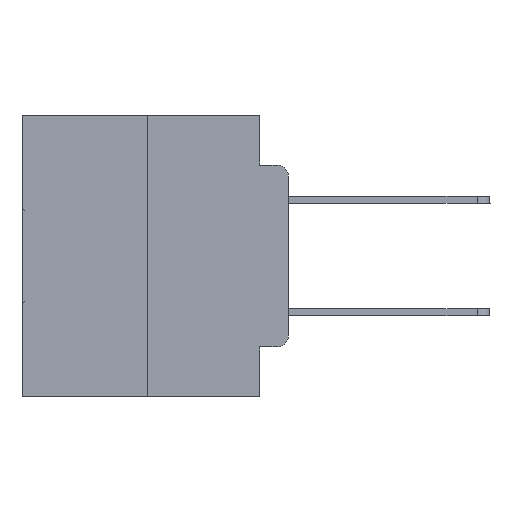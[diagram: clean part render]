
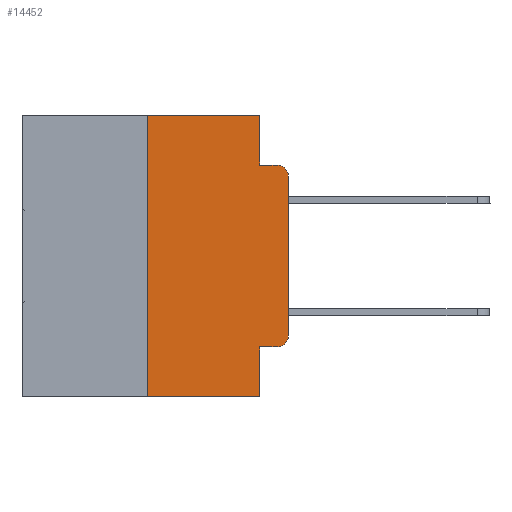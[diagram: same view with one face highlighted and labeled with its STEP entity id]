
A CAD part, left-side view. The second image highlights one B-rep face of the part: STEP entity #14452.
In plain terms, the highlighted planar face has unit normal (-1, 0, 0).
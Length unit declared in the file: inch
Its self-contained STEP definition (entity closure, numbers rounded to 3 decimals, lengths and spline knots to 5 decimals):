
#887 = VECTOR ( 'NONE', #26429, 39.37008 ) ;
#1592 = CARTESIAN_POINT ( 'NONE',  ( 0., 0.051, -0.0885 ) ) ;
#2279 = DIRECTION ( 'NONE',  ( 0., 0., -1. ) ) ;
#2426 = DIRECTION ( 'NONE',  ( 0., 0., 1. ) ) ;
#2488 = VERTEX_POINT ( 'NONE', #21263 ) ;
#2617 = AXIS2_PLACEMENT_3D ( 'NONE', #30579, #9293, #16163 ) ;
#2816 = ORIENTED_EDGE ( 'NONE', *, *, #7497, .T. ) ;
#3326 = CARTESIAN_POINT ( 'NONE',  ( 0., 0.25, 0. ) ) ;
#3633 = VERTEX_POINT ( 'NONE', #7026 ) ;
#3906 = VERTEX_POINT ( 'NONE', #6482 ) ;
#5116 = EDGE_CURVE ( 'NONE', #2488, #24602, #30207, .T. ) ;
#5413 = DIRECTION ( 'NONE',  ( 0., 0., 1. ) ) ;
#5499 = VERTEX_POINT ( 'NONE', #8828 ) ;
#6482 = CARTESIAN_POINT ( 'NONE',  ( 0., 0.051, -0.4115 ) ) ;
#6509 = VECTOR ( 'NONE', #29588, 39.37008 ) ;
#7026 = CARTESIAN_POINT ( 'NONE',  ( 0., 0., -0.1085 ) ) ;
#7497 = EDGE_CURVE ( 'NONE', #2488, #29429, #12756, .T. ) ;
#7513 = CARTESIAN_POINT ( 'NONE',  ( 0., 0.051, -0.5 ) ) ;
#8701 = AXIS2_PLACEMENT_3D ( 'NONE', #16530, #21446, #2279 ) ;
#8759 = CARTESIAN_POINT ( 'NONE',  ( 0., 0.051, -0.0885 ) ) ;
#8828 = CARTESIAN_POINT ( 'NONE',  ( 0., 0., -0.3915 ) ) ;
#9293 = DIRECTION ( 'NONE',  ( 1., 0., 0. ) ) ;
#9789 = VECTOR ( 'NONE', #5413, 39.37008 ) ;
#10036 = ORIENTED_EDGE ( 'NONE', *, *, #5116, .F. ) ;
#10191 = VERTEX_POINT ( 'NONE', #1592 ) ;
#10495 = VECTOR ( 'NONE', #16469, 39.37008 ) ;
#10659 = VERTEX_POINT ( 'NONE', #20377 ) ;
#10724 = LINE ( 'NONE', #8759, #15228 ) ;
#12074 = DIRECTION ( 'NONE',  ( 0., 0., -1. ) ) ;
#12575 = LINE ( 'NONE', #21474, #887 ) ;
#12756 = LINE ( 'NONE', #31098, #10495 ) ;
#12823 = CARTESIAN_POINT ( 'NONE',  ( 0., 0.473, 0. ) ) ;
#12904 = LINE ( 'NONE', #12823, #6509 ) ;
#12958 = EDGE_CURVE ( 'NONE', #24602, #29509, #12904, .T. ) ;
#13052 = DIRECTION ( 'NONE',  ( 0., 0., -1. ) ) ;
#13186 = FACE_OUTER_BOUND ( 'NONE', #17552, .T. ) ;
#13832 = EDGE_CURVE ( 'NONE', #14276, #5499, #26831, .T. ) ;
#14136 = VECTOR ( 'NONE', #13052, 39.37008 ) ;
#14276 = VERTEX_POINT ( 'NONE', #27922 ) ;
#14342 = CARTESIAN_POINT ( 'NONE',  ( 0., 0.25, 0. ) ) ;
#14365 = DIRECTION ( 'NONE',  ( 0., 0., -1. ) ) ;
#14381 = DIRECTION ( 'NONE',  ( -1., 0., 0. ) ) ;
#14452 = ADVANCED_FACE ( 'NONE', ( #13186 ), #30798, .F. ) ;
#14622 = EDGE_CURVE ( 'NONE', #5499, #3633, #23374, .T. ) ;
#15228 = VECTOR ( 'NONE', #23198, 39.37008 ) ;
#15565 = ORIENTED_EDGE ( 'NONE', *, *, #13832, .T. ) ;
#16163 = DIRECTION ( 'NONE',  ( 0., 0., -1. ) ) ;
#16469 = DIRECTION ( 'NONE',  ( 0., -1., 0. ) ) ;
#16530 = CARTESIAN_POINT ( 'NONE',  ( 0., 0.02, -0.1085 ) ) ;
#17552 = EDGE_LOOP ( 'NONE', ( #24741, #29118, #23249, #23381, #22470, #10036, #2816, #29877, #19213, #15565 ) ) ;
#17888 = LINE ( 'NONE', #29405, #14136 ) ;
#19213 = ORIENTED_EDGE ( 'NONE', *, *, #25050, .T. ) ;
#20377 = CARTESIAN_POINT ( 'NONE',  ( 0., 0.02, -0.0885 ) ) ;
#21263 = CARTESIAN_POINT ( 'NONE',  ( 0., 0.25, -0.5 ) ) ;
#21446 = DIRECTION ( 'NONE',  ( -1., 0., 0. ) ) ;
#21474 = CARTESIAN_POINT ( 'NONE',  ( 0., 0.051, -0.4115 ) ) ;
#21711 = EDGE_CURVE ( 'NONE', #29509, #10191, #31122, .T. ) ;
#21881 = EDGE_CURVE ( 'NONE', #3906, #29429, #17888, .T. ) ;
#22470 = ORIENTED_EDGE ( 'NONE', *, *, #12958, .F. ) ;
#23011 = EDGE_CURVE ( 'NONE', #3633, #10659, #29554, .T. ) ;
#23023 = VECTOR ( 'NONE', #2426, 39.37008 ) ;
#23198 = DIRECTION ( 'NONE',  ( 0., -1., 0. ) ) ;
#23249 = ORIENTED_EDGE ( 'NONE', *, *, #24182, .F. ) ;
#23374 = LINE ( 'NONE', #31200, #9789 ) ;
#23381 = ORIENTED_EDGE ( 'NONE', *, *, #21711, .F. ) ;
#23590 = VECTOR ( 'NONE', #14365, 39.37008 ) ;
#23960 = CARTESIAN_POINT ( 'NONE',  ( 0., 0.02, -0.3915 ) ) ;
#24046 = CARTESIAN_POINT ( 'NONE',  ( 0., 0.051, 0. ) ) ;
#24182 = EDGE_CURVE ( 'NONE', #10191, #10659, #10724, .T. ) ;
#24589 = CARTESIAN_POINT ( 'NONE',  ( 0., 0.051, 0. ) ) ;
#24602 = VERTEX_POINT ( 'NONE', #3326 ) ;
#24608 = AXIS2_PLACEMENT_3D ( 'NONE', #23960, #14381, #12074 ) ;
#24741 = ORIENTED_EDGE ( 'NONE', *, *, #14622, .T. ) ;
#25050 = EDGE_CURVE ( 'NONE', #3906, #14276, #12575, .T. ) ;
#26429 = DIRECTION ( 'NONE',  ( 0., -1., 0. ) ) ;
#26831 = CIRCLE ( 'NONE', #24608, 0.02 ) ;
#27922 = CARTESIAN_POINT ( 'NONE',  ( 0., 0.02, -0.4115 ) ) ;
#29118 = ORIENTED_EDGE ( 'NONE', *, *, #23011, .T. ) ;
#29405 = CARTESIAN_POINT ( 'NONE',  ( 0., 0.051, 0. ) ) ;
#29429 = VERTEX_POINT ( 'NONE', #7513 ) ;
#29509 = VERTEX_POINT ( 'NONE', #24589 ) ;
#29554 = CIRCLE ( 'NONE', #8701, 0.02 ) ;
#29588 = DIRECTION ( 'NONE',  ( 0., -1., 0. ) ) ;
#29877 = ORIENTED_EDGE ( 'NONE', *, *, #21881, .F. ) ;
#30207 = LINE ( 'NONE', #14342, #23023 ) ;
#30579 = CARTESIAN_POINT ( 'NONE',  ( 0., 0.473, 0. ) ) ;
#30798 = PLANE ( 'NONE',  #2617 ) ;
#31098 = CARTESIAN_POINT ( 'NONE',  ( 0., 0.473, -0.5 ) ) ;
#31122 = LINE ( 'NONE', #24046, #23590 ) ;
#31200 = CARTESIAN_POINT ( 'NONE',  ( 0., 0., 0. ) ) ;
